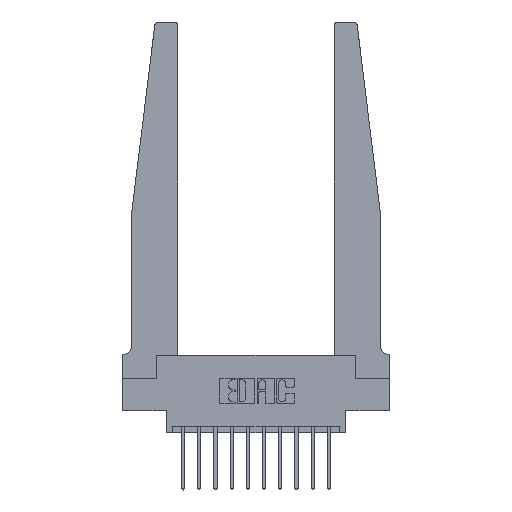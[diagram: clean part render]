
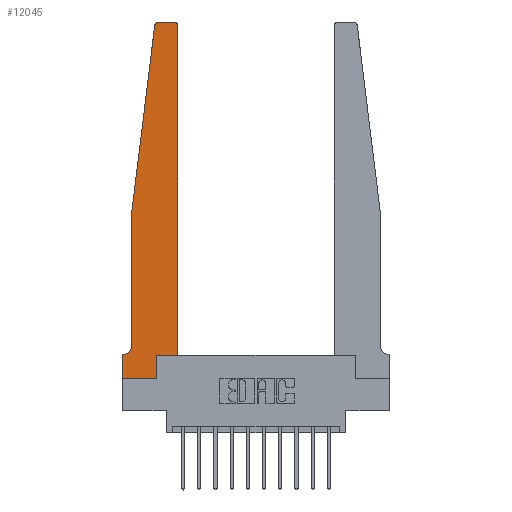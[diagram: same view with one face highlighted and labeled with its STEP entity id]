
A CAD part, top view. The second image highlights one B-rep face of the part: STEP entity #12045.
In plain terms, the highlighted planar face has unit normal (0, 0, 1).
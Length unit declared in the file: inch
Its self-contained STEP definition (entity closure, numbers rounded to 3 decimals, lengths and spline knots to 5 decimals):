
#107 = DIRECTION ( 'NONE',  ( -1., 0., 0. ) ) ;
#136 = ORIENTED_EDGE ( 'NONE', *, *, #4214, .T. ) ;
#138 = CARTESIAN_POINT ( 'NONE',  ( 0., 0., 0.37 ) ) ;
#236 = CARTESIAN_POINT ( 'NONE',  ( 0.395, 2.72, 0.37 ) ) ;
#311 = CIRCLE ( 'NONE', #15117, 0.03 ) ;
#333 = CARTESIAN_POINT ( 'NONE',  ( 0.27653, 2.75, 0.37 ) ) ;
#358 = VERTEX_POINT ( 'NONE', #14699 ) ;
#664 = ORIENTED_EDGE ( 'NONE', *, *, #7788, .T. ) ;
#708 = DIRECTION ( 'NONE',  ( -0.122, -0.992, 0. ) ) ;
#788 = CARTESIAN_POINT ( 'NONE',  ( 0.2605, 0., 0.37 ) ) ;
#1291 = CARTESIAN_POINT ( 'NONE',  ( 0., 0.1875, 0.37 ) ) ;
#1452 = DIRECTION ( 'NONE',  ( 1., 0., 0. ) ) ;
#1476 = LINE ( 'NONE', #4435, #7972 ) ;
#1525 = LINE ( 'NONE', #138, #4790 ) ;
#1553 = CARTESIAN_POINT ( 'NONE',  ( 0.425, 2.72, 0.37 ) ) ;
#1640 = CARTESIAN_POINT ( 'NONE',  ( 0., 0., 0.37 ) ) ;
#1645 = DIRECTION ( 'NONE',  ( 1., 0., 0. ) ) ;
#1854 = CARTESIAN_POINT ( 'NONE',  ( 0.2605, 0.18, 0.37 ) ) ;
#2126 = LINE ( 'NONE', #8952, #15133 ) ;
#2228 = ORIENTED_EDGE ( 'NONE', *, *, #10179, .T. ) ;
#2372 = CIRCLE ( 'NONE', #15468, 0.03 ) ;
#2436 = DIRECTION ( 'NONE',  ( 0., -1., 0. ) ) ;
#2497 = DIRECTION ( 'NONE',  ( 1., 0., 0. ) ) ;
#2754 = CIRCLE ( 'NONE', #8943, 0.05 ) ;
#2799 = CARTESIAN_POINT ( 'NONE',  ( 0., 0., 0.37 ) ) ;
#2943 = ORIENTED_EDGE ( 'NONE', *, *, #15225, .T. ) ;
#3054 = VECTOR ( 'NONE', #11568, 39.37008 ) ;
#3065 = DIRECTION ( 'NONE',  ( 0., 1., 0. ) ) ;
#3436 = LINE ( 'NONE', #4224, #3054 ) ;
#3611 = EDGE_CURVE ( 'NONE', #9590, #14235, #2754, .T. ) ;
#3699 = EDGE_CURVE ( 'NONE', #12209, #11282, #2372, .T. ) ;
#3862 = CARTESIAN_POINT ( 'NONE',  ( 0.27653, 2.72, 0.37 ) ) ;
#4161 = ORIENTED_EDGE ( 'NONE', *, *, #10989, .T. ) ;
#4214 = EDGE_CURVE ( 'NONE', #12315, #9124, #1525, .T. ) ;
#4224 = CARTESIAN_POINT ( 'NONE',  ( 0.425, 0.18, 0.37 ) ) ;
#4349 = ORIENTED_EDGE ( 'NONE', *, *, #3611, .T. ) ;
#4435 = CARTESIAN_POINT ( 'NONE',  ( 0.25, 2.75, 0.37 ) ) ;
#4700 = VECTOR ( 'NONE', #708, 39.37008 ) ;
#4790 = VECTOR ( 'NONE', #6218, 39.37008 ) ;
#5114 = DIRECTION ( 'NONE',  ( 1., 0., 0. ) ) ;
#5681 = LINE ( 'NONE', #1854, #11804 ) ;
#5702 = EDGE_LOOP ( 'NONE', ( #11733, #10827, #8258, #2943, #4349, #664, #136, #2228, #11491, #4161, #6535, #8714 ) ) ;
#5742 = CARTESIAN_POINT ( 'NONE',  ( 0.24675, 2.72367, 0.37 ) ) ;
#5863 = VERTEX_POINT ( 'NONE', #13318 ) ;
#6218 = DIRECTION ( 'NONE',  ( 0., -1., 0. ) ) ;
#6535 = ORIENTED_EDGE ( 'NONE', *, *, #11658, .T. ) ;
#6692 = EDGE_CURVE ( 'NONE', #6804, #358, #5681, .T. ) ;
#6799 = CARTESIAN_POINT ( 'NONE',  ( 0.065, 1.25, 0.37 ) ) ;
#6804 = VERTEX_POINT ( 'NONE', #788 ) ;
#7316 = CARTESIAN_POINT ( 'NONE',  ( 0.065, 0.2375, 0.37 ) ) ;
#7390 = DIRECTION ( 'NONE',  ( 0., 0., -1. ) ) ;
#7629 = EDGE_CURVE ( 'NONE', #12193, #11453, #311, .T. ) ;
#7788 = EDGE_CURVE ( 'NONE', #14235, #12315, #13857, .T. ) ;
#7934 = LINE ( 'NONE', #6799, #4700 ) ;
#7972 = VECTOR ( 'NONE', #12992, 39.37008 ) ;
#8026 = EDGE_CURVE ( 'NONE', #11282, #10566, #7934, .T. ) ;
#8258 = ORIENTED_EDGE ( 'NONE', *, *, #8026, .T. ) ;
#8614 = AXIS2_PLACEMENT_3D ( 'NONE', #1291, #9836, #2497 ) ;
#8714 = ORIENTED_EDGE ( 'NONE', *, *, #7629, .T. ) ;
#8767 = DIRECTION ( 'NONE',  ( 0., 0., 1. ) ) ;
#8821 = VECTOR ( 'NONE', #11382, 39.37008 ) ;
#8943 = AXIS2_PLACEMENT_3D ( 'NONE', #14718, #7390, #107 ) ;
#8952 = CARTESIAN_POINT ( 'NONE',  ( 0.425, 0.18, 0.37 ) ) ;
#9124 = VERTEX_POINT ( 'NONE', #1640 ) ;
#9590 = VERTEX_POINT ( 'NONE', #7316 ) ;
#9787 = CARTESIAN_POINT ( 'NONE',  ( 0.065, 1.25, 0.37 ) ) ;
#9836 = DIRECTION ( 'NONE',  ( 0., 0., 1. ) ) ;
#10179 = EDGE_CURVE ( 'NONE', #9124, #6804, #11700, .T. ) ;
#10566 = VERTEX_POINT ( 'NONE', #13190 ) ;
#10631 = LINE ( 'NONE', #9787, #13880 ) ;
#10827 = ORIENTED_EDGE ( 'NONE', *, *, #3699, .T. ) ;
#10970 = CARTESIAN_POINT ( 'NONE',  ( 0.395, 2.75, 0.37 ) ) ;
#10989 = EDGE_CURVE ( 'NONE', #358, #5863, #2126, .T. ) ;
#11014 = PLANE ( 'NONE',  #8614 ) ;
#11282 = VERTEX_POINT ( 'NONE', #5742 ) ;
#11382 = DIRECTION ( 'NONE',  ( 1., 0., 0. ) ) ;
#11453 = VERTEX_POINT ( 'NONE', #10970 ) ;
#11491 = ORIENTED_EDGE ( 'NONE', *, *, #6692, .T. ) ;
#11568 = DIRECTION ( 'NONE',  ( 0., 1., 0. ) ) ;
#11583 = CARTESIAN_POINT ( 'NONE',  ( 0.015, 0.1875, 0.37 ) ) ;
#11658 = EDGE_CURVE ( 'NONE', #5863, #12193, #3436, .T. ) ;
#11700 = LINE ( 'NONE', #2799, #8821 ) ;
#11733 = ORIENTED_EDGE ( 'NONE', *, *, #14957, .T. ) ;
#11804 = VECTOR ( 'NONE', #3065, 39.37008 ) ;
#12045 = ADVANCED_FACE ( 'NONE', ( #13579 ), #11014, .T. ) ;
#12193 = VERTEX_POINT ( 'NONE', #1553 ) ;
#12209 = VERTEX_POINT ( 'NONE', #333 ) ;
#12315 = VERTEX_POINT ( 'NONE', #13935 ) ;
#12439 = DIRECTION ( 'NONE',  ( 0., 0., 1. ) ) ;
#12471 = CARTESIAN_POINT ( 'NONE',  ( 0.065, 0.1875, 0.37 ) ) ;
#12992 = DIRECTION ( 'NONE',  ( -1., 0., 0. ) ) ;
#13190 = CARTESIAN_POINT ( 'NONE',  ( 0.065, 1.25, 0.37 ) ) ;
#13318 = CARTESIAN_POINT ( 'NONE',  ( 0.425, 0.18, 0.37 ) ) ;
#13579 = FACE_OUTER_BOUND ( 'NONE', #5702, .T. ) ;
#13857 = LINE ( 'NONE', #12471, #14242 ) ;
#13880 = VECTOR ( 'NONE', #2436, 39.37008 ) ;
#13935 = CARTESIAN_POINT ( 'NONE',  ( 0., 0.1875, 0.37 ) ) ;
#14235 = VERTEX_POINT ( 'NONE', #11583 ) ;
#14242 = VECTOR ( 'NONE', #14917, 39.37008 ) ;
#14699 = CARTESIAN_POINT ( 'NONE',  ( 0.2605, 0.18, 0.37 ) ) ;
#14718 = CARTESIAN_POINT ( 'NONE',  ( 0.015, 0.2375, 0.37 ) ) ;
#14917 = DIRECTION ( 'NONE',  ( -1., 0., 0. ) ) ;
#14957 = EDGE_CURVE ( 'NONE', #11453, #12209, #1476, .T. ) ;
#15117 = AXIS2_PLACEMENT_3D ( 'NONE', #236, #8767, #1452 ) ;
#15133 = VECTOR ( 'NONE', #1645, 39.37008 ) ;
#15225 = EDGE_CURVE ( 'NONE', #10566, #9590, #10631, .T. ) ;
#15468 = AXIS2_PLACEMENT_3D ( 'NONE', #3862, #12439, #5114 ) ;
